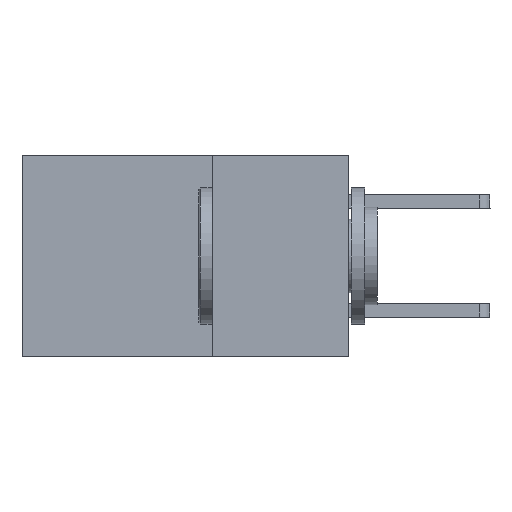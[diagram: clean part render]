
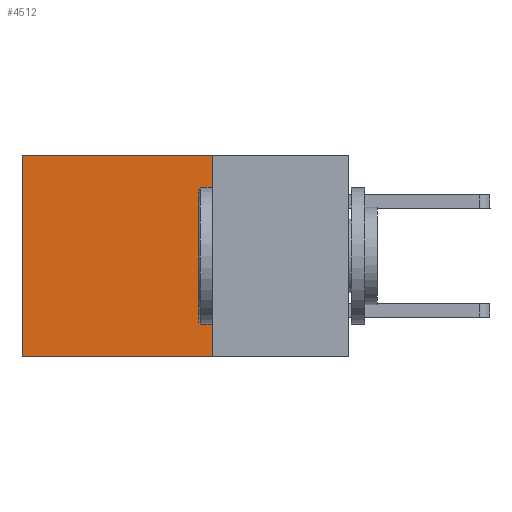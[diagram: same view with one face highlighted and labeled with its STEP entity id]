
A CAD part, left-side view. The second image highlights one B-rep face of the part: STEP entity #4512.
In plain terms, the highlighted planar face has unit normal (-1, 0, 0).
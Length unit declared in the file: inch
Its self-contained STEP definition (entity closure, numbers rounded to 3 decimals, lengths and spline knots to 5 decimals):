
#47 = PLANE ( 'NONE',  #5883 ) ;
#56 = VERTEX_POINT ( 'NONE', #1834 ) ;
#186 = VECTOR ( 'NONE', #9460, 39.37008 ) ;
#453 = CARTESIAN_POINT ( 'NONE',  ( 0.2615, 0.25, 0. ) ) ;
#551 = LINE ( 'NONE', #453, #186 ) ;
#1024 = LINE ( 'NONE', #3340, #4110 ) ;
#1285 = CARTESIAN_POINT ( 'NONE',  ( 0.2615, 0.25, -0.37 ) ) ;
#1822 = DIRECTION ( 'NONE',  ( 0., 1., 0. ) ) ;
#1834 = CARTESIAN_POINT ( 'NONE',  ( 0.2615, 0.25, 0. ) ) ;
#1997 = ORIENTED_EDGE ( 'NONE', *, *, #2105, .F. ) ;
#2105 = EDGE_CURVE ( 'NONE', #56, #8729, #8815, .T. ) ;
#2873 = CARTESIAN_POINT ( 'NONE',  ( 0.2615, 0.6, 0. ) ) ;
#3340 = CARTESIAN_POINT ( 'NONE',  ( 0.2615, 0.25, -0.37 ) ) ;
#3722 = DIRECTION ( 'NONE',  ( 0., 0., -1. ) ) ;
#3883 = CARTESIAN_POINT ( 'NONE',  ( 0.2615, 0.25, -0.37 ) ) ;
#4110 = VECTOR ( 'NONE', #1822, 39.37008 ) ;
#4512 = ADVANCED_FACE ( 'NONE', ( #8402 ), #47, .F. ) ;
#5371 = VECTOR ( 'NONE', #3722, 39.37008 ) ;
#5407 = EDGE_CURVE ( 'NONE', #56, #9206, #551, .T. ) ;
#5434 = EDGE_LOOP ( 'NONE', ( #6720, #6648, #1997, #6499 ) ) ;
#5883 = AXIS2_PLACEMENT_3D ( 'NONE', #3883, #8972, #9159 ) ;
#5887 = VERTEX_POINT ( 'NONE', #8688 ) ;
#5951 = CARTESIAN_POINT ( 'NONE',  ( 0.2615, 0.25, -0.37 ) ) ;
#6359 = LINE ( 'NONE', #7183, #7147 ) ;
#6499 = ORIENTED_EDGE ( 'NONE', *, *, #5407, .T. ) ;
#6520 = DIRECTION ( 'NONE',  ( 0., 0., -1. ) ) ;
#6546 = EDGE_CURVE ( 'NONE', #9206, #5887, #6359, .T. ) ;
#6648 = ORIENTED_EDGE ( 'NONE', *, *, #8146, .F. ) ;
#6720 = ORIENTED_EDGE ( 'NONE', *, *, #6546, .T. ) ;
#7147 = VECTOR ( 'NONE', #6520, 39.37008 ) ;
#7183 = CARTESIAN_POINT ( 'NONE',  ( 0.2615, 0.6, -0.37 ) ) ;
#8146 = EDGE_CURVE ( 'NONE', #8729, #5887, #1024, .T. ) ;
#8402 = FACE_OUTER_BOUND ( 'NONE', #5434, .T. ) ;
#8688 = CARTESIAN_POINT ( 'NONE',  ( 0.2615, 0.6, -0.37 ) ) ;
#8729 = VERTEX_POINT ( 'NONE', #1285 ) ;
#8815 = LINE ( 'NONE', #5951, #5371 ) ;
#8972 = DIRECTION ( 'NONE',  ( 1., 0., 0. ) ) ;
#9159 = DIRECTION ( 'NONE',  ( 0., 0., -1. ) ) ;
#9206 = VERTEX_POINT ( 'NONE', #2873 ) ;
#9460 = DIRECTION ( 'NONE',  ( 0., 1., 0. ) ) ;
